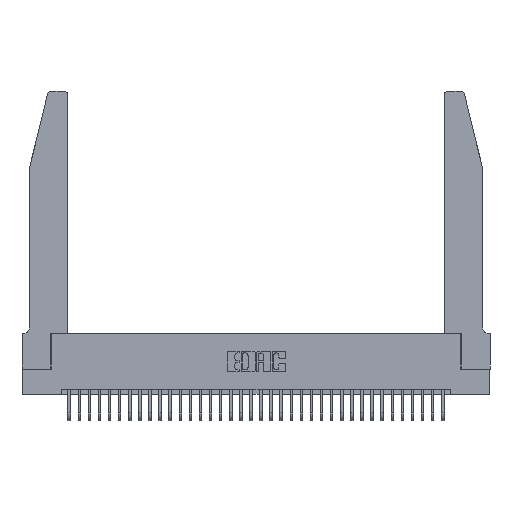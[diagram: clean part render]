
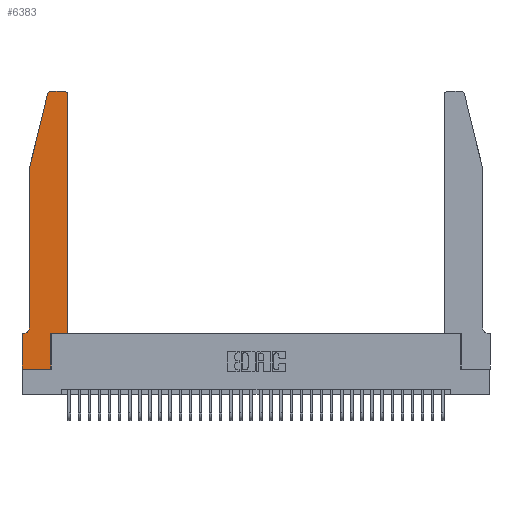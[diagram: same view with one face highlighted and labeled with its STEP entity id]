
A CAD part, top view. The second image highlights one B-rep face of the part: STEP entity #6383.
In plain terms, the highlighted planar face has unit normal (0, 0, 1).
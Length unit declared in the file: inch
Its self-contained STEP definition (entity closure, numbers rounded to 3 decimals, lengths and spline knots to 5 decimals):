
#98 = LINE ( 'NONE', #8922, #28907 ) ;
#859 = VERTEX_POINT ( 'NONE', #21808 ) ;
#1819 = ORIENTED_EDGE ( 'NONE', *, *, #13968, .T. ) ;
#2271 = EDGE_CURVE ( 'NONE', #9254, #19586, #35884, .T. ) ;
#2429 = EDGE_CURVE ( 'NONE', #31908, #28613, #22489, .T. ) ;
#2676 = LINE ( 'NONE', #9357, #5341 ) ;
#2819 = VERTEX_POINT ( 'NONE', #18851 ) ;
#3120 = CARTESIAN_POINT ( 'NONE',  ( 0.4205, 2.75, 0.37 ) ) ;
#3452 = VECTOR ( 'NONE', #33469, 39.37008 ) ;
#3580 = CARTESIAN_POINT ( 'NONE',  ( 0.25487, 2.72718, 0.37 ) ) ;
#3677 = CARTESIAN_POINT ( 'NONE',  ( 0., 0.35, 0.37 ) ) ;
#3754 = VERTEX_POINT ( 'NONE', #11032 ) ;
#3800 = DIRECTION ( 'NONE',  ( 1., 0., 0. ) ) ;
#4661 = DIRECTION ( 'NONE',  ( 1., 0., 0. ) ) ;
#4692 = AXIS2_PLACEMENT_3D ( 'NONE', #3677, #22903, #3800 ) ;
#4725 = ORIENTED_EDGE ( 'NONE', *, *, #8098, .T. ) ;
#4862 = VECTOR ( 'NONE', #13530, 39.37008 ) ;
#5218 = VERTEX_POINT ( 'NONE', #3120 ) ;
#5341 = VECTOR ( 'NONE', #35453, 39.37008 ) ;
#5786 = DIRECTION ( 'NONE',  ( -1., 0., 0. ) ) ;
#6172 = DIRECTION ( 'NONE',  ( 1., 0., 0. ) ) ;
#6383 = ADVANCED_FACE ( 'NONE', ( #29596 ), #14356, .T. ) ;
#7692 = ORIENTED_EDGE ( 'NONE', *, *, #24413, .T. ) ;
#8098 = EDGE_CURVE ( 'NONE', #2819, #32837, #36643, .T. ) ;
#8588 = CIRCLE ( 'NONE', #26610, 0.03 ) ;
#8922 = CARTESIAN_POINT ( 'NONE',  ( 0., 0., 0.37 ) ) ;
#9254 = VERTEX_POINT ( 'NONE', #20226 ) ;
#9266 = LINE ( 'NONE', #10191, #4862 ) ;
#9357 = CARTESIAN_POINT ( 'NONE',  ( 0.2605, 2.75, 0.37 ) ) ;
#9558 = EDGE_CURVE ( 'NONE', #28812, #3754, #28087, .T. ) ;
#9650 = ORIENTED_EDGE ( 'NONE', *, *, #9952, .T. ) ;
#9952 = EDGE_CURVE ( 'NONE', #24157, #5218, #8588, .T. ) ;
#10191 = CARTESIAN_POINT ( 'NONE',  ( 0.4505, 0.35, 0.37 ) ) ;
#10258 = ORIENTED_EDGE ( 'NONE', *, *, #2429, .T. ) ;
#10924 = CARTESIAN_POINT ( 'NONE',  ( 0.2865, 0.35, 0.37 ) ) ;
#11032 = CARTESIAN_POINT ( 'NONE',  ( 0.2865, 0.35, 0.37 ) ) ;
#13530 = DIRECTION ( 'NONE',  ( 1., 0., 0. ) ) ;
#13968 = EDGE_CURVE ( 'NONE', #3754, #15720, #9266, .T. ) ;
#14003 = DIRECTION ( 'NONE',  ( 0., 0., 1. ) ) ;
#14079 = DIRECTION ( 'NONE',  ( 0., 0., -1. ) ) ;
#14356 = PLANE ( 'NONE',  #4692 ) ;
#14367 = DIRECTION ( 'NONE',  ( -1., 0., 0. ) ) ;
#14492 = DIRECTION ( 'NONE',  ( 1., 0., 0. ) ) ;
#14738 = CARTESIAN_POINT ( 'NONE',  ( 0.0055, 0.35, 0.37 ) ) ;
#15173 = CARTESIAN_POINT ( 'NONE',  ( 0.284, 2.72, 0.37 ) ) ;
#15335 = CARTESIAN_POINT ( 'NONE',  ( 0.4505, 0.35, 0.37 ) ) ;
#15720 = VERTEX_POINT ( 'NONE', #15335 ) ;
#15887 = LINE ( 'NONE', #27578, #3452 ) ;
#16601 = ORIENTED_EDGE ( 'NONE', *, *, #26526, .T. ) ;
#17026 = CARTESIAN_POINT ( 'NONE',  ( 0., 0.35, 0.37 ) ) ;
#17156 = VECTOR ( 'NONE', #14367, 39.37008 ) ;
#18296 = ORIENTED_EDGE ( 'NONE', *, *, #26650, .T. ) ;
#18625 = CARTESIAN_POINT ( 'NONE',  ( 0.0755, 2., 0.37 ) ) ;
#18757 = DIRECTION ( 'NONE',  ( 0., 0., 1. ) ) ;
#18851 = CARTESIAN_POINT ( 'NONE',  ( 0.0755, 2., 0.37 ) ) ;
#19586 = VERTEX_POINT ( 'NONE', #3580 ) ;
#19642 = VECTOR ( 'NONE', #31750, 39.37008 ) ;
#20226 = CARTESIAN_POINT ( 'NONE',  ( 0.284, 2.75, 0.37 ) ) ;
#20483 = ORIENTED_EDGE ( 'NONE', *, *, #31414, .T. ) ;
#20996 = CARTESIAN_POINT ( 'NONE',  ( 0.4205, 2.72, 0.37 ) ) ;
#21808 = CARTESIAN_POINT ( 'NONE',  ( 0., 0., 0.37 ) ) ;
#22285 = CARTESIAN_POINT ( 'NONE',  ( 0.0055, 0.42, 0.37 ) ) ;
#22368 = VECTOR ( 'NONE', #26324, 39.37008 ) ;
#22489 = LINE ( 'NONE', #28585, #17156 ) ;
#22903 = DIRECTION ( 'NONE',  ( 0., 0., 1. ) ) ;
#22986 = ORIENTED_EDGE ( 'NONE', *, *, #31269, .T. ) ;
#24157 = VERTEX_POINT ( 'NONE', #33167 ) ;
#24413 = EDGE_CURVE ( 'NONE', #15720, #24157, #28084, .T. ) ;
#25458 = AXIS2_PLACEMENT_3D ( 'NONE', #15173, #14003, #6172 ) ;
#26324 = DIRECTION ( 'NONE',  ( 0., 1., 0. ) ) ;
#26526 = EDGE_CURVE ( 'NONE', #28613, #859, #15887, .T. ) ;
#26602 = ORIENTED_EDGE ( 'NONE', *, *, #9558, .T. ) ;
#26610 = AXIS2_PLACEMENT_3D ( 'NONE', #20996, #18757, #4661 ) ;
#26650 = EDGE_CURVE ( 'NONE', #32837, #31908, #36780, .T. ) ;
#26712 = DIRECTION ( 'NONE',  ( 0., -1., 0. ) ) ;
#26773 = CARTESIAN_POINT ( 'NONE',  ( 0.2865, 0., 0.37 ) ) ;
#27028 = ORIENTED_EDGE ( 'NONE', *, *, #29302, .T. ) ;
#27067 = DIRECTION ( 'NONE',  ( -0.239, -0.971, 0. ) ) ;
#27305 = VECTOR ( 'NONE', #26712, 39.37008 ) ;
#27460 = VECTOR ( 'NONE', #27067, 39.37008 ) ;
#27578 = CARTESIAN_POINT ( 'NONE',  ( 0., 0., 0.37 ) ) ;
#28084 = LINE ( 'NONE', #28730, #19642 ) ;
#28087 = LINE ( 'NONE', #10924, #22368 ) ;
#28585 = CARTESIAN_POINT ( 'NONE',  ( 0.0755, 0.35, 0.37 ) ) ;
#28613 = VERTEX_POINT ( 'NONE', #17026 ) ;
#28730 = CARTESIAN_POINT ( 'NONE',  ( 0.4505, 0.35, 0.37 ) ) ;
#28812 = VERTEX_POINT ( 'NONE', #26773 ) ;
#28907 = VECTOR ( 'NONE', #14492, 39.37008 ) ;
#29302 = EDGE_CURVE ( 'NONE', #859, #28812, #98, .T. ) ;
#29596 = FACE_OUTER_BOUND ( 'NONE', #31578, .T. ) ;
#30632 = CARTESIAN_POINT ( 'NONE',  ( 0.0755, 0.42, 0.37 ) ) ;
#31269 = EDGE_CURVE ( 'NONE', #5218, #9254, #2676, .T. ) ;
#31414 = EDGE_CURVE ( 'NONE', #19586, #2819, #36396, .T. ) ;
#31578 = EDGE_LOOP ( 'NONE', ( #22986, #34148, #20483, #4725, #18296, #10258, #16601, #27028, #26602, #1819, #7692, #9650 ) ) ;
#31750 = DIRECTION ( 'NONE',  ( 0., 1., 0. ) ) ;
#31908 = VERTEX_POINT ( 'NONE', #14738 ) ;
#32592 = CARTESIAN_POINT ( 'NONE',  ( 0.0755, 2., 0.37 ) ) ;
#32837 = VERTEX_POINT ( 'NONE', #30632 ) ;
#33167 = CARTESIAN_POINT ( 'NONE',  ( 0.4505, 2.72, 0.37 ) ) ;
#33469 = DIRECTION ( 'NONE',  ( 0., -1., 0. ) ) ;
#34148 = ORIENTED_EDGE ( 'NONE', *, *, #2271, .T. ) ;
#35453 = DIRECTION ( 'NONE',  ( -1., 0., 0. ) ) ;
#35884 = CIRCLE ( 'NONE', #25458, 0.03 ) ;
#36063 = AXIS2_PLACEMENT_3D ( 'NONE', #22285, #14079, #5786 ) ;
#36396 = LINE ( 'NONE', #18625, #27460 ) ;
#36643 = LINE ( 'NONE', #32592, #27305 ) ;
#36780 = CIRCLE ( 'NONE', #36063, 0.07 ) ;
